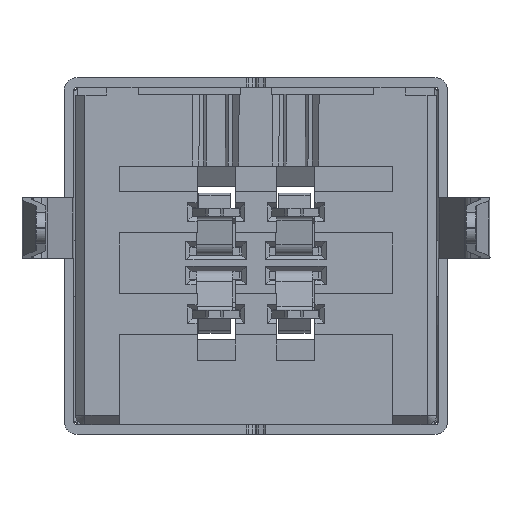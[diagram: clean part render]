
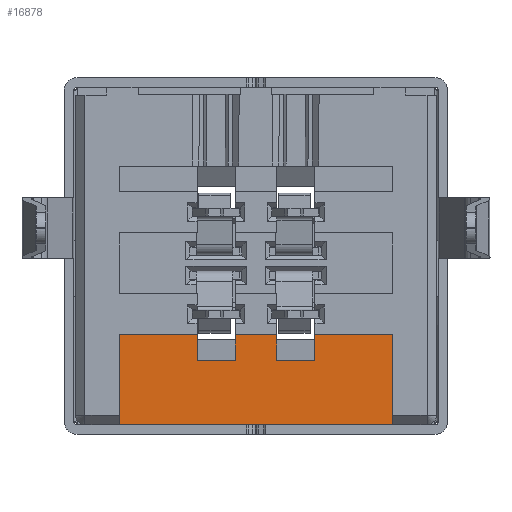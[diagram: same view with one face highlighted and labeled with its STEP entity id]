
A CAD part, front view. The second image highlights one B-rep face of the part: STEP entity #16878.
In plain terms, the highlighted face is planar.
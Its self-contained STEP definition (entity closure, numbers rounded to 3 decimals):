
#36 = LINE ( 'NONE', #7573, #4972 ) ;
#567 = VECTOR ( 'NONE', #6236, 1000. ) ;
#726 = VECTOR ( 'NONE', #6804, 1000. ) ;
#968 = EDGE_LOOP ( 'NONE', ( #24332, #20119, #23914, #1553, #7163, #14141, #8101, #7217, #21701, #12199, #10227, #11135 ) ) ;
#1211 = CARTESIAN_POINT ( 'NONE',  ( 30.302, 24.139, -10.325 ) ) ;
#1450 = VERTEX_POINT ( 'NONE', #1211 ) ;
#1551 = VECTOR ( 'NONE', #16349, 1000. ) ;
#1553 = ORIENTED_EDGE ( 'NONE', *, *, #4270, .T. ) ;
#1665 = EDGE_CURVE ( 'NONE', #3705, #17803, #20693, .T. ) ;
#1831 = VECTOR ( 'NONE', #7118, 1000. ) ;
#2185 = VERTEX_POINT ( 'NONE', #20661 ) ;
#2289 = CARTESIAN_POINT ( 'NONE',  ( 30.302, 24.94, -6.025 ) ) ;
#2336 = CARTESIAN_POINT ( 'NONE',  ( 30.302, 24.139, -5.375 ) ) ;
#2619 = LINE ( 'NONE', #12241, #22471 ) ;
#3063 = DIRECTION ( 'NONE',  ( 0., 1., 0. ) ) ;
#3339 = CARTESIAN_POINT ( 'NONE',  ( 30.302, 18.677, -10.497 ) ) ;
#3388 = VERTEX_POINT ( 'NONE', #24141 ) ;
#3412 = EDGE_CURVE ( 'NONE', #1450, #12942, #7235, .T. ) ;
#3574 = VERTEX_POINT ( 'NONE', #20909 ) ;
#3705 = VERTEX_POINT ( 'NONE', #13639 ) ;
#3991 = CARTESIAN_POINT ( 'NONE',  ( 30.302, 24.94, -6.675 ) ) ;
#4270 = EDGE_CURVE ( 'NONE', #17623, #10810, #22701, .T. ) ;
#4972 = VECTOR ( 'NONE', #5604, 1000. ) ;
#5033 = CARTESIAN_POINT ( 'NONE',  ( 30.302, 25.552, -10.325 ) ) ;
#5082 = VERTEX_POINT ( 'NONE', #11511 ) ;
#5604 = DIRECTION ( 'NONE',  ( 0., 0., -1. ) ) ;
#5636 = VECTOR ( 'NONE', #16918, 1000. ) ;
#5781 = VECTOR ( 'NONE', #11485, 1000. ) ;
#6134 = EDGE_CURVE ( 'NONE', #5082, #3388, #2619, .T. ) ;
#6227 = VECTOR ( 'NONE', #24159, 1000. ) ;
#6236 = DIRECTION ( 'NONE',  ( 0., -1., 0. ) ) ;
#6711 = LINE ( 'NONE', #19657, #1551 ) ;
#6804 = DIRECTION ( 'NONE',  ( 0., -1., 0. ) ) ;
#7118 = DIRECTION ( 'NONE',  ( 0., 1., 0. ) ) ;
#7163 = ORIENTED_EDGE ( 'NONE', *, *, #21638, .T. ) ;
#7217 = ORIENTED_EDGE ( 'NONE', *, *, #15408, .T. ) ;
#7235 = LINE ( 'NONE', #5033, #1831 ) ;
#7421 = CARTESIAN_POINT ( 'NONE',  ( 30.302, 24.94, -6.025 ) ) ;
#7472 = EDGE_CURVE ( 'NONE', #19801, #3705, #22588, .T. ) ;
#7573 = CARTESIAN_POINT ( 'NONE',  ( 30.302, 24.139, -6.025 ) ) ;
#7893 = LINE ( 'NONE', #9388, #5636 ) ;
#8085 = LINE ( 'NONE', #23369, #567 ) ;
#8101 = ORIENTED_EDGE ( 'NONE', *, *, #1665, .T. ) ;
#9013 = DIRECTION ( 'NONE',  ( 0., 1., 0. ) ) ;
#9388 = CARTESIAN_POINT ( 'NONE',  ( 30.302, 26.965, -6.025 ) ) ;
#9628 = VECTOR ( 'NONE', #3063, 1000. ) ;
#10227 = ORIENTED_EDGE ( 'NONE', *, *, #3412, .T. ) ;
#10300 = CARTESIAN_POINT ( 'NONE',  ( 30.302, 26.965, -1.725 ) ) ;
#10481 = AXIS2_PLACEMENT_3D ( 'NONE', #3339, #10855, #9013 ) ;
#10810 = VERTEX_POINT ( 'NONE', #21862 ) ;
#10855 = DIRECTION ( 'NONE',  ( 1., 0., 0. ) ) ;
#11135 = ORIENTED_EDGE ( 'NONE', *, *, #13487, .F. ) ;
#11485 = DIRECTION ( 'NONE',  ( 0., 0., -1. ) ) ;
#11511 = CARTESIAN_POINT ( 'NONE',  ( 30.302, 24.139, -1.725 ) ) ;
#11907 = DIRECTION ( 'NONE',  ( 0., 0., -1. ) ) ;
#12105 = CARTESIAN_POINT ( 'NONE',  ( 30.302, 22.902, -5.375 ) ) ;
#12199 = ORIENTED_EDGE ( 'NONE', *, *, #16788, .T. ) ;
#12241 = CARTESIAN_POINT ( 'NONE',  ( 30.302, 24.139, -6.025 ) ) ;
#12942 = VERTEX_POINT ( 'NONE', #17569 ) ;
#13487 = EDGE_CURVE ( 'NONE', #15428, #12942, #7893, .T. ) ;
#13639 = CARTESIAN_POINT ( 'NONE',  ( 30.302, 24.139, -6.675 ) ) ;
#14141 = ORIENTED_EDGE ( 'NONE', *, *, #7472, .T. ) ;
#14652 = LINE ( 'NONE', #16622, #9628 ) ;
#15141 = EDGE_CURVE ( 'NONE', #3388, #17623, #14652, .T. ) ;
#15338 = EDGE_CURVE ( 'NONE', #15428, #5082, #8085, .T. ) ;
#15408 = EDGE_CURVE ( 'NONE', #17803, #2185, #21397, .T. ) ;
#15428 = VERTEX_POINT ( 'NONE', #10300 ) ;
#15999 = CARTESIAN_POINT ( 'NONE',  ( 30.302, 24.94, -4.175 ) ) ;
#16065 = PLANE ( 'NONE',  #10481 ) ;
#16349 = DIRECTION ( 'NONE',  ( 0., -1., 0. ) ) ;
#16622 = CARTESIAN_POINT ( 'NONE',  ( 30.302, 22.902, -4.175 ) ) ;
#16788 = EDGE_CURVE ( 'NONE', #3574, #1450, #36, .T. ) ;
#16878 = ADVANCED_FACE ( 'NONE', ( #20226 ), #16065, .T. ) ;
#16918 = DIRECTION ( 'NONE',  ( 0., 0., -1. ) ) ;
#17569 = CARTESIAN_POINT ( 'NONE',  ( 30.302, 26.965, -10.325 ) ) ;
#17623 = VERTEX_POINT ( 'NONE', #15999 ) ;
#17803 = VERTEX_POINT ( 'NONE', #3991 ) ;
#17965 = VECTOR ( 'NONE', #22816, 1000. ) ;
#18026 = LINE ( 'NONE', #12105, #726 ) ;
#19657 = CARTESIAN_POINT ( 'NONE',  ( 30.302, 22.902, -7.875 ) ) ;
#19801 = VERTEX_POINT ( 'NONE', #2336 ) ;
#20119 = ORIENTED_EDGE ( 'NONE', *, *, #6134, .T. ) ;
#20226 = FACE_OUTER_BOUND ( 'NONE', #968, .T. ) ;
#20661 = CARTESIAN_POINT ( 'NONE',  ( 30.302, 24.94, -7.875 ) ) ;
#20693 = LINE ( 'NONE', #23927, #6227 ) ;
#20909 = CARTESIAN_POINT ( 'NONE',  ( 30.302, 24.139, -7.875 ) ) ;
#21370 = DIRECTION ( 'NONE',  ( 0., 0., -1. ) ) ;
#21397 = LINE ( 'NONE', #2289, #21444 ) ;
#21444 = VECTOR ( 'NONE', #11907, 1000. ) ;
#21638 = EDGE_CURVE ( 'NONE', #10810, #19801, #18026, .T. ) ;
#21701 = ORIENTED_EDGE ( 'NONE', *, *, #22458, .T. ) ;
#21862 = CARTESIAN_POINT ( 'NONE',  ( 30.302, 24.94, -5.375 ) ) ;
#22458 = EDGE_CURVE ( 'NONE', #2185, #3574, #6711, .T. ) ;
#22471 = VECTOR ( 'NONE', #21370, 1000. ) ;
#22588 = LINE ( 'NONE', #24000, #5781 ) ;
#22701 = LINE ( 'NONE', #7421, #17965 ) ;
#22816 = DIRECTION ( 'NONE',  ( 0., 0., -1. ) ) ;
#23369 = CARTESIAN_POINT ( 'NONE',  ( 30.302, 22.902, -1.725 ) ) ;
#23914 = ORIENTED_EDGE ( 'NONE', *, *, #15141, .T. ) ;
#23927 = CARTESIAN_POINT ( 'NONE',  ( 30.302, 22.902, -6.675 ) ) ;
#24000 = CARTESIAN_POINT ( 'NONE',  ( 30.302, 24.139, -6.025 ) ) ;
#24141 = CARTESIAN_POINT ( 'NONE',  ( 30.302, 24.139, -4.175 ) ) ;
#24159 = DIRECTION ( 'NONE',  ( 0., 1., 0. ) ) ;
#24332 = ORIENTED_EDGE ( 'NONE', *, *, #15338, .T. ) ;
